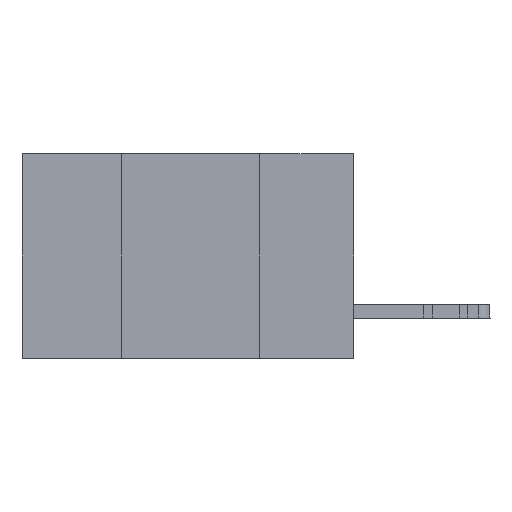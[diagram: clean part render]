
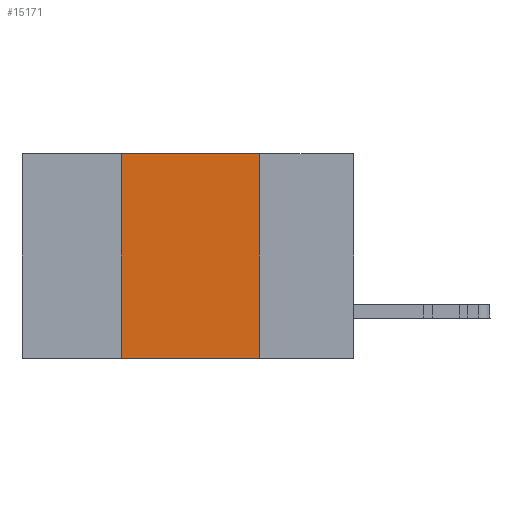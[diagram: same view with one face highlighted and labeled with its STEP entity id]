
A CAD part, left-side view. The second image highlights one B-rep face of the part: STEP entity #15171.
In plain terms, the highlighted planar face has unit normal (-1, 0, 0).
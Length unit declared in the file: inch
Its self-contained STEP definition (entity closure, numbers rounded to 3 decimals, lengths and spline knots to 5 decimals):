
#2608 = DIRECTION ( 'NONE',  ( 0., -1., 0. ) ) ;
#2990 = DIRECTION ( 'NONE',  ( 0., 0., -1. ) ) ;
#3280 = CARTESIAN_POINT ( 'NONE',  ( 0., 0.42, -0.37 ) ) ;
#3821 = EDGE_CURVE ( 'NONE', #31884, #33990, #41473, .T. ) ;
#4527 = VECTOR ( 'NONE', #35926, 39.37008 ) ;
#5935 = DIRECTION ( 'NONE',  ( 0., 0., -1. ) ) ;
#8305 = AXIS2_PLACEMENT_3D ( 'NONE', #35253, #24709, #2990 ) ;
#8969 = VECTOR ( 'NONE', #12646, 39.37008 ) ;
#9716 = VECTOR ( 'NONE', #2608, 39.37008 ) ;
#10265 = PLANE ( 'NONE',  #8305 ) ;
#11476 = ORIENTED_EDGE ( 'NONE', *, *, #3821, .T. ) ;
#12646 = DIRECTION ( 'NONE',  ( 0., 0., 1. ) ) ;
#15102 = EDGE_CURVE ( 'NONE', #15559, #16448, #26773, .T. ) ;
#15171 = ADVANCED_FACE ( 'NONE', ( #26226 ), #10265, .F. ) ;
#15559 = VERTEX_POINT ( 'NONE', #19457 ) ;
#16448 = VERTEX_POINT ( 'NONE', #32414 ) ;
#18264 = VECTOR ( 'NONE', #5935, 39.37008 ) ;
#18687 = LINE ( 'NONE', #30752, #8969 ) ;
#19210 = ORIENTED_EDGE ( 'NONE', *, *, #15102, .F. ) ;
#19457 = CARTESIAN_POINT ( 'NONE',  ( 0., 0.42, 0. ) ) ;
#21561 = CARTESIAN_POINT ( 'NONE',  ( 0., 0.17, -0.37 ) ) ;
#24709 = DIRECTION ( 'NONE',  ( 1., 0., 0. ) ) ;
#25005 = LINE ( 'NONE', #34852, #18264 ) ;
#26226 = FACE_OUTER_BOUND ( 'NONE', #27987, .T. ) ;
#26773 = LINE ( 'NONE', #36876, #9716 ) ;
#27987 = EDGE_LOOP ( 'NONE', ( #44234, #19210, #29599, #11476 ) ) ;
#28251 = EDGE_CURVE ( 'NONE', #16448, #33990, #25005, .T. ) ;
#29599 = ORIENTED_EDGE ( 'NONE', *, *, #37259, .F. ) ;
#30752 = CARTESIAN_POINT ( 'NONE',  ( 0., 0.42, 0. ) ) ;
#31884 = VERTEX_POINT ( 'NONE', #3280 ) ;
#32414 = CARTESIAN_POINT ( 'NONE',  ( 0., 0.17, 0. ) ) ;
#33990 = VERTEX_POINT ( 'NONE', #21561 ) ;
#34852 = CARTESIAN_POINT ( 'NONE',  ( 0., 0.17, 0. ) ) ;
#35253 = CARTESIAN_POINT ( 'NONE',  ( 0., 0.6, 0. ) ) ;
#35926 = DIRECTION ( 'NONE',  ( 0., -1., 0. ) ) ;
#36876 = CARTESIAN_POINT ( 'NONE',  ( 0., 0.6, 0. ) ) ;
#37259 = EDGE_CURVE ( 'NONE', #31884, #15559, #18687, .T. ) ;
#39270 = CARTESIAN_POINT ( 'NONE',  ( 0., 0.6, -0.37 ) ) ;
#41473 = LINE ( 'NONE', #39270, #4527 ) ;
#44234 = ORIENTED_EDGE ( 'NONE', *, *, #28251, .F. ) ;
